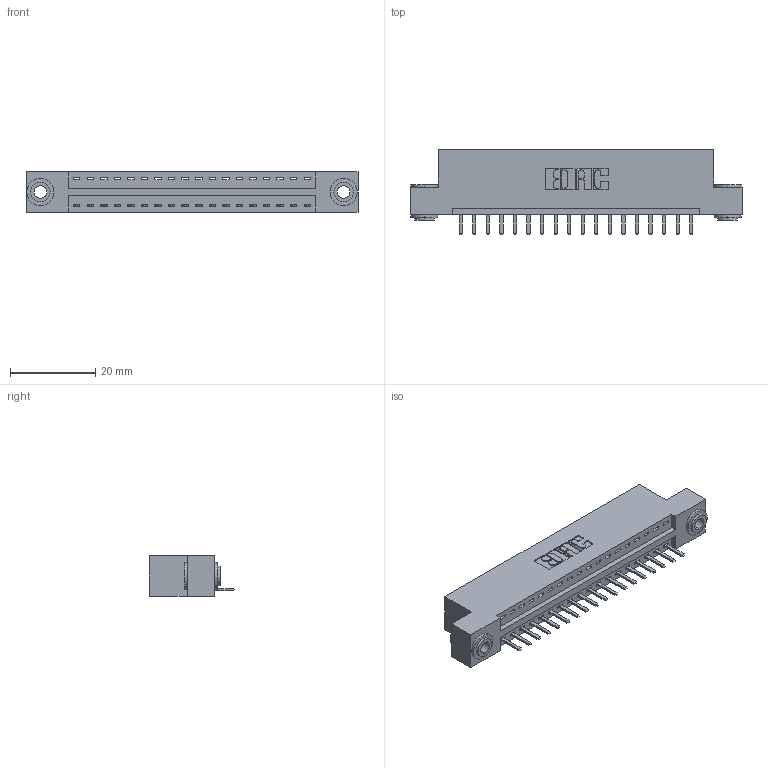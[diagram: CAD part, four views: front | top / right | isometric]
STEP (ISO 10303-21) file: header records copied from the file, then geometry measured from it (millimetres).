
FILE_DESCRIPTION (( 'STEP AP203' ), '1' );
FILE_NAME ('396-018-520-103.STEP', '2019-10-26T19:23:08', ( '' ), ( '' ), 'SwSTEP 2.0', 'SolidWorks 2016', '' );
FILE_SCHEMA (( 'CONFIG_CONTROL_DESIGN' ));
Length unit declared in the file: inch
Products named in the file (4): 346 Part_Flush Mounting Lugs - 0.156 Dia-TH; 345-250-002_345-250-002-102; 396-018-520-103; 345-292-001_345-293-120
Assembly tree (21 placements, depth 2):
  396-018-520-103
    346 Part_Flush Mounting Lugs - 0.156 Dia-TH
    345-292-001_345-293-120  x18
    345-250-002_345-250-002-102  x2
Bounding box: 77.72 x 20.02 x 9.4 mm (x, y, z)
Volume: 7242.2 mm3; surface area: 8839.1 mm2
Topology: 21 solids, 21 shells, 1276 faces, 3717 edges, 2426 vertices
Faces by surface type: plane 842, cylinder 426, cone 8
Entity records: 15166 total; most frequent: CARTESIAN_POINT 2597, ORIENTED_EDGE 2530, DIRECTION 2339, EDGE_CURVE 1265, LINE 1033, VECTOR 1033, VERTEX_POINT 838, AXIS2_PLACEMENT_3D 653
